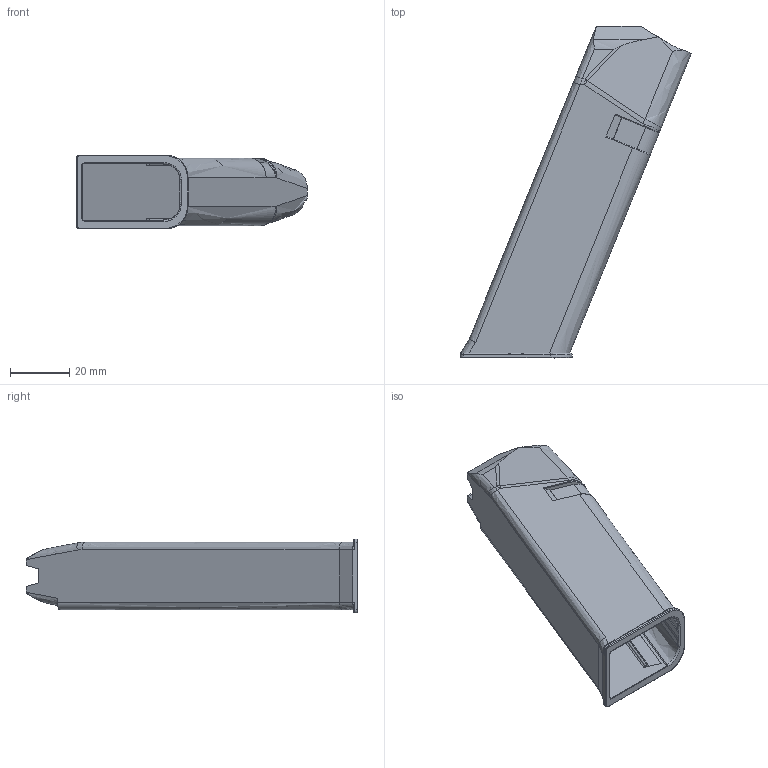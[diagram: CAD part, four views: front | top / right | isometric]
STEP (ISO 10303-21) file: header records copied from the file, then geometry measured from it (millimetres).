
FILE_DESCRIPTION(/* description */ (''),/* implementation_level */ '2;1');
FILE_NAME(/* name */ 'Menendez Mag Body V1.61.stp',/* time_stamp */ '2019-06-27T23:09:29-05:00',/* author */ ('johne'),/* organization */ (''),/* preprocessor_version */ 'ST-DEVELOPER v16.13',/* originating_system */ 'Autodesk Inventor 2018',/* authorisation */ '');
FILE_SCHEMA (('AUTOMOTIVE_DESIGN { 1 0 10303 214 3 1 1 }'));
Length unit declared in the file: inch
Products named in the file (1): Menendez Mag Body V1.61
Bounding box: 77.74 x 111.88 x 24.87 mm (x, y, z)
Volume: 20184.3 mm3; surface area: 23889 mm2
Topology: 1 solids, 5 shells, 400 faces, 1122 edges, 791 vertices
Faces by surface type: plane 228, bspline 133, cylinder 37, cone 2
Entity records: 15400 total; most frequent: CARTESIAN_POINT 5500, ORIENTED_EDGE 2110, DIRECTION 1777, EDGE_CURVE 1054, LINE 673, VECTOR 673, VERTEX_POINT 663, AXIS2_PLACEMENT_3D 552
